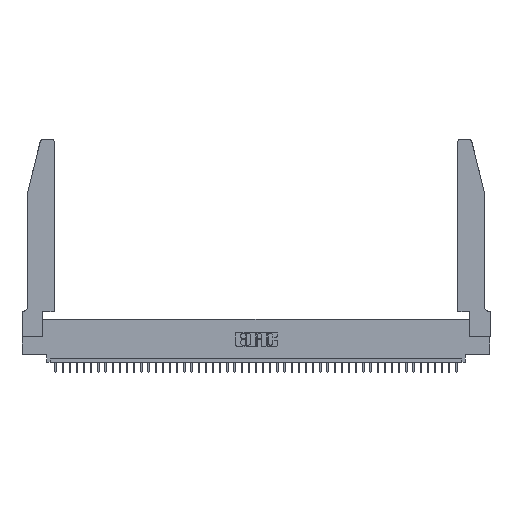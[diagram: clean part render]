
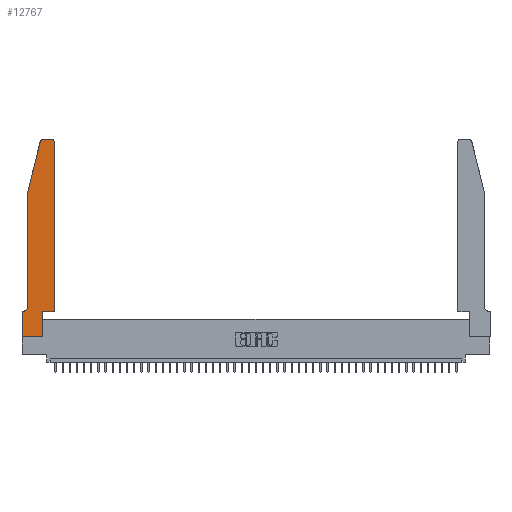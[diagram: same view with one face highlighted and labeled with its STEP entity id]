
A CAD part, top view. The second image highlights one B-rep face of the part: STEP entity #12767.
In plain terms, the highlighted planar face has unit normal (0, 0, 1).
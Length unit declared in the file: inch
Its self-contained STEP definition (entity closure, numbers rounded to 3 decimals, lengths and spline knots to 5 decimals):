
#153 = EDGE_CURVE ( 'NONE', #28533, #23909, #14224, .T. ) ;
#685 = DIRECTION ( 'NONE',  ( 0., 0., 1. ) ) ;
#742 = CIRCLE ( 'NONE', #6720, 0.03 ) ;
#909 = CARTESIAN_POINT ( 'NONE',  ( 0., 0.35, 0.37 ) ) ;
#2291 = DIRECTION ( 'NONE',  ( 1., 0., 0. ) ) ;
#3249 = ORIENTED_EDGE ( 'NONE', *, *, #7904, .T. ) ;
#3310 = CARTESIAN_POINT ( 'NONE',  ( 0.0755, 2., 0.37 ) ) ;
#4304 = VERTEX_POINT ( 'NONE', #15358 ) ;
#4652 = CIRCLE ( 'NONE', #10606, 0.03 ) ;
#4728 = EDGE_LOOP ( 'NONE', ( #22251, #17854, #12771, #27983, #14500, #34201, #3249, #34727, #43649, #43214, #36004, #34844 ) ) ;
#4730 = CARTESIAN_POINT ( 'NONE',  ( 0., 0., 0.37 ) ) ;
#6087 = DIRECTION ( 'NONE',  ( 0., 0., 1. ) ) ;
#6720 = AXIS2_PLACEMENT_3D ( 'NONE', #16527, #6087, #37406 ) ;
#7904 = EDGE_CURVE ( 'NONE', #36251, #19058, #36487, .T. ) ;
#7910 = EDGE_CURVE ( 'NONE', #34189, #16235, #31774, .T. ) ;
#8356 = CARTESIAN_POINT ( 'NONE',  ( 0.4505, 0.35, 0.37 ) ) ;
#9403 = CARTESIAN_POINT ( 'NONE',  ( 0.2865, 0.35, 0.37 ) ) ;
#10159 = VERTEX_POINT ( 'NONE', #40755 ) ;
#10606 = AXIS2_PLACEMENT_3D ( 'NONE', #24341, #23639, #2291 ) ;
#10789 = DIRECTION ( 'NONE',  ( -1., 0., 0. ) ) ;
#10882 = VECTOR ( 'NONE', #14003, 39.37008 ) ;
#11127 = CARTESIAN_POINT ( 'NONE',  ( 0.0755, 2., 0.37 ) ) ;
#12022 = VECTOR ( 'NONE', #16288, 39.37008 ) ;
#12705 = VECTOR ( 'NONE', #29049, 39.37008 ) ;
#12767 = ADVANCED_FACE ( 'NONE', ( #21795 ), #32694, .T. ) ;
#12771 = ORIENTED_EDGE ( 'NONE', *, *, #32662, .T. ) ;
#14003 = DIRECTION ( 'NONE',  ( 0., -1., 0. ) ) ;
#14224 = LINE ( 'NONE', #35979, #12705 ) ;
#14500 = ORIENTED_EDGE ( 'NONE', *, *, #7910, .T. ) ;
#14759 = CARTESIAN_POINT ( 'NONE',  ( 0.4505, 0.35, 0.37 ) ) ;
#14862 = LINE ( 'NONE', #8356, #39123 ) ;
#15202 = DIRECTION ( 'NONE',  ( 0., 1., 0. ) ) ;
#15358 = CARTESIAN_POINT ( 'NONE',  ( 0.2865, 0., 0.37 ) ) ;
#16235 = VERTEX_POINT ( 'NONE', #30951 ) ;
#16288 = DIRECTION ( 'NONE',  ( -0.239, -0.971, 0. ) ) ;
#16394 = DIRECTION ( 'NONE',  ( 1., 0., 0. ) ) ;
#16527 = CARTESIAN_POINT ( 'NONE',  ( 0.284, 2.72, 0.37 ) ) ;
#17319 = LINE ( 'NONE', #38185, #18316 ) ;
#17569 = VERTEX_POINT ( 'NONE', #26250 ) ;
#17854 = ORIENTED_EDGE ( 'NONE', *, *, #19359, .T. ) ;
#18316 = VECTOR ( 'NONE', #16394, 39.37008 ) ;
#18951 = VERTEX_POINT ( 'NONE', #9403 ) ;
#19058 = VERTEX_POINT ( 'NONE', #28200 ) ;
#19359 = EDGE_CURVE ( 'NONE', #23909, #17569, #742, .T. ) ;
#19924 = VECTOR ( 'NONE', #22557, 39.37008 ) ;
#21795 = FACE_OUTER_BOUND ( 'NONE', #4728, .T. ) ;
#21800 = CARTESIAN_POINT ( 'NONE',  ( 0.0755, 0.42, 0.37 ) ) ;
#22251 = ORIENTED_EDGE ( 'NONE', *, *, #153, .T. ) ;
#22557 = DIRECTION ( 'NONE',  ( 0., 1., 0. ) ) ;
#23639 = DIRECTION ( 'NONE',  ( 0., 0., 1. ) ) ;
#23909 = VERTEX_POINT ( 'NONE', #34002 ) ;
#24341 = CARTESIAN_POINT ( 'NONE',  ( 0.4205, 2.72, 0.37 ) ) ;
#24410 = EDGE_CURVE ( 'NONE', #33333, #34189, #27691, .T. ) ;
#24463 = EDGE_CURVE ( 'NONE', #16235, #36251, #31634, .T. ) ;
#25171 = DIRECTION ( 'NONE',  ( 0., 0., -1. ) ) ;
#25758 = DIRECTION ( 'NONE',  ( 1., 0., 0. ) ) ;
#26095 = EDGE_CURVE ( 'NONE', #18951, #10159, #14862, .T. ) ;
#26250 = CARTESIAN_POINT ( 'NONE',  ( 0.25487, 2.72718, 0.37 ) ) ;
#26286 = LINE ( 'NONE', #40874, #12022 ) ;
#26552 = AXIS2_PLACEMENT_3D ( 'NONE', #39978, #25171, #10789 ) ;
#26920 = EDGE_CURVE ( 'NONE', #4304, #18951, #43187, .T. ) ;
#27691 = LINE ( 'NONE', #3310, #10882 ) ;
#27983 = ORIENTED_EDGE ( 'NONE', *, *, #24410, .T. ) ;
#28200 = CARTESIAN_POINT ( 'NONE',  ( 0., 0., 0.37 ) ) ;
#28533 = VERTEX_POINT ( 'NONE', #28809 ) ;
#28809 = CARTESIAN_POINT ( 'NONE',  ( 0.4205, 2.75, 0.37 ) ) ;
#28852 = CARTESIAN_POINT ( 'NONE',  ( 0.2865, 0.35, 0.37 ) ) ;
#29049 = DIRECTION ( 'NONE',  ( -1., 0., 0. ) ) ;
#30439 = VECTOR ( 'NONE', #15202, 39.37008 ) ;
#30857 = EDGE_CURVE ( 'NONE', #10159, #42317, #43254, .T. ) ;
#30951 = CARTESIAN_POINT ( 'NONE',  ( 0.0055, 0.35, 0.37 ) ) ;
#31634 = LINE ( 'NONE', #41593, #41226 ) ;
#31774 = CIRCLE ( 'NONE', #26552, 0.07 ) ;
#32662 = EDGE_CURVE ( 'NONE', #17569, #33333, #26286, .T. ) ;
#32694 = PLANE ( 'NONE',  #45654 ) ;
#32760 = CARTESIAN_POINT ( 'NONE',  ( 0.4505, 2.72, 0.37 ) ) ;
#32806 = DIRECTION ( 'NONE',  ( 0., -1., 0. ) ) ;
#33333 = VERTEX_POINT ( 'NONE', #11127 ) ;
#34002 = CARTESIAN_POINT ( 'NONE',  ( 0.284, 2.75, 0.37 ) ) ;
#34189 = VERTEX_POINT ( 'NONE', #21800 ) ;
#34201 = ORIENTED_EDGE ( 'NONE', *, *, #24463, .T. ) ;
#34403 = DIRECTION ( 'NONE',  ( -1., 0., 0. ) ) ;
#34727 = ORIENTED_EDGE ( 'NONE', *, *, #44736, .T. ) ;
#34844 = ORIENTED_EDGE ( 'NONE', *, *, #37278, .T. ) ;
#35924 = DIRECTION ( 'NONE',  ( 1., 0., 0. ) ) ;
#35979 = CARTESIAN_POINT ( 'NONE',  ( 0.2605, 2.75, 0.37 ) ) ;
#36004 = ORIENTED_EDGE ( 'NONE', *, *, #30857, .T. ) ;
#36170 = VECTOR ( 'NONE', #32806, 39.37008 ) ;
#36251 = VERTEX_POINT ( 'NONE', #40226 ) ;
#36487 = LINE ( 'NONE', #4730, #36170 ) ;
#37278 = EDGE_CURVE ( 'NONE', #42317, #28533, #4652, .T. ) ;
#37406 = DIRECTION ( 'NONE',  ( 1., 0., 0. ) ) ;
#38185 = CARTESIAN_POINT ( 'NONE',  ( 0., 0., 0.37 ) ) ;
#39123 = VECTOR ( 'NONE', #25758, 39.37008 ) ;
#39978 = CARTESIAN_POINT ( 'NONE',  ( 0.0055, 0.42, 0.37 ) ) ;
#40226 = CARTESIAN_POINT ( 'NONE',  ( 0., 0.35, 0.37 ) ) ;
#40755 = CARTESIAN_POINT ( 'NONE',  ( 0.4505, 0.35, 0.37 ) ) ;
#40874 = CARTESIAN_POINT ( 'NONE',  ( 0.0755, 2., 0.37 ) ) ;
#41226 = VECTOR ( 'NONE', #34403, 39.37008 ) ;
#41593 = CARTESIAN_POINT ( 'NONE',  ( 0.0755, 0.35, 0.37 ) ) ;
#42317 = VERTEX_POINT ( 'NONE', #32760 ) ;
#43187 = LINE ( 'NONE', #28852, #19924 ) ;
#43214 = ORIENTED_EDGE ( 'NONE', *, *, #26095, .T. ) ;
#43254 = LINE ( 'NONE', #14759, #30439 ) ;
#43649 = ORIENTED_EDGE ( 'NONE', *, *, #26920, .T. ) ;
#44736 = EDGE_CURVE ( 'NONE', #19058, #4304, #17319, .T. ) ;
#45654 = AXIS2_PLACEMENT_3D ( 'NONE', #909, #685, #35924 ) ;
